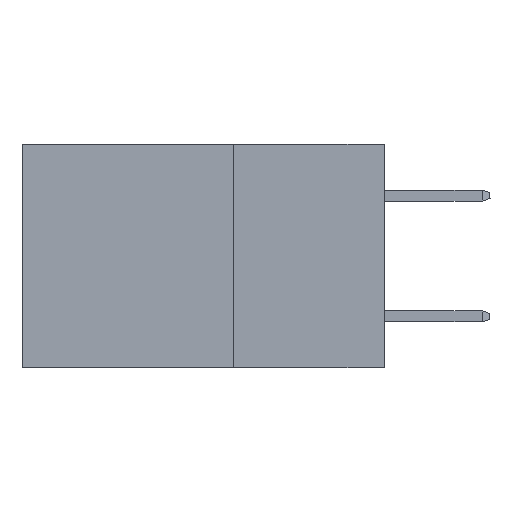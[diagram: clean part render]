
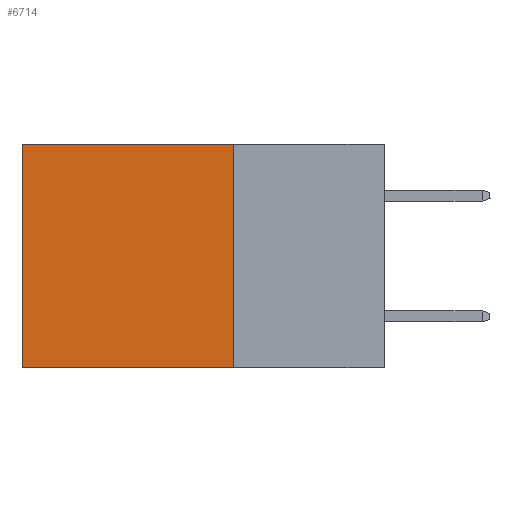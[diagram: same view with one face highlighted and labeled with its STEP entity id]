
A CAD part, left-side view. The second image highlights one B-rep face of the part: STEP entity #6714.
In plain terms, the highlighted planar face has unit normal (-1, 0, 0).
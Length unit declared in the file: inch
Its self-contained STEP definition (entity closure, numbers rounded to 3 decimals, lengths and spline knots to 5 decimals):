
#1019 = LINE ( 'NONE', #1693, #11804 ) ;
#1693 = CARTESIAN_POINT ( 'NONE',  ( 0.298, 0.25, -0.37 ) ) ;
#1700 = CARTESIAN_POINT ( 'NONE',  ( 0.298, 0.25, 0. ) ) ;
#2309 = DIRECTION ( 'NONE',  ( 1., 0., 0. ) ) ;
#3394 = VERTEX_POINT ( 'NONE', #7946 ) ;
#4358 = DIRECTION ( 'NONE',  ( 0., 0., -1. ) ) ;
#4794 = VECTOR ( 'NONE', #5563, 39.37008 ) ;
#5341 = VECTOR ( 'NONE', #8683, 39.37008 ) ;
#5563 = DIRECTION ( 'NONE',  ( 0., 0., -1. ) ) ;
#5700 = EDGE_CURVE ( 'NONE', #6472, #3394, #18338, .T. ) ;
#6137 = CARTESIAN_POINT ( 'NONE',  ( 0.298, 0.25, -0.37 ) ) ;
#6292 = CARTESIAN_POINT ( 'NONE',  ( 0.298, 0.6, 0. ) ) ;
#6388 = ORIENTED_EDGE ( 'NONE', *, *, #12717, .F. ) ;
#6472 = VERTEX_POINT ( 'NONE', #6292 ) ;
#6546 = DIRECTION ( 'NONE',  ( 0., 0., -1. ) ) ;
#6593 = VECTOR ( 'NONE', #4358, 39.37008 ) ;
#6714 = ADVANCED_FACE ( 'NONE', ( #7460 ), #10868, .F. ) ;
#7234 = CARTESIAN_POINT ( 'NONE',  ( 0.298, 0.25, 0. ) ) ;
#7239 = VERTEX_POINT ( 'NONE', #6137 ) ;
#7460 = FACE_OUTER_BOUND ( 'NONE', #9712, .T. ) ;
#7594 = AXIS2_PLACEMENT_3D ( 'NONE', #18423, #2309, #6546 ) ;
#7946 = CARTESIAN_POINT ( 'NONE',  ( 0.298, 0.6, -0.37 ) ) ;
#8539 = EDGE_CURVE ( 'NONE', #15580, #6472, #18913, .T. ) ;
#8683 = DIRECTION ( 'NONE',  ( 0., 1., 0. ) ) ;
#9172 = DIRECTION ( 'NONE',  ( 0., 1., 0. ) ) ;
#9712 = EDGE_LOOP ( 'NONE', ( #9832, #6388, #17833, #17265 ) ) ;
#9832 = ORIENTED_EDGE ( 'NONE', *, *, #5700, .T. ) ;
#10868 = PLANE ( 'NONE',  #7594 ) ;
#11804 = VECTOR ( 'NONE', #9172, 39.37008 ) ;
#12717 = EDGE_CURVE ( 'NONE', #7239, #3394, #1019, .T. ) ;
#12824 = LINE ( 'NONE', #7234, #6593 ) ;
#12889 = CARTESIAN_POINT ( 'NONE',  ( 0.298, 0.25, 0. ) ) ;
#14246 = CARTESIAN_POINT ( 'NONE',  ( 0.298, 0.6, 0. ) ) ;
#15580 = VERTEX_POINT ( 'NONE', #1700 ) ;
#16838 = EDGE_CURVE ( 'NONE', #15580, #7239, #12824, .T. ) ;
#17265 = ORIENTED_EDGE ( 'NONE', *, *, #8539, .T. ) ;
#17833 = ORIENTED_EDGE ( 'NONE', *, *, #16838, .F. ) ;
#18338 = LINE ( 'NONE', #14246, #4794 ) ;
#18423 = CARTESIAN_POINT ( 'NONE',  ( 0.298, 0.25, 0. ) ) ;
#18913 = LINE ( 'NONE', #12889, #5341 ) ;
